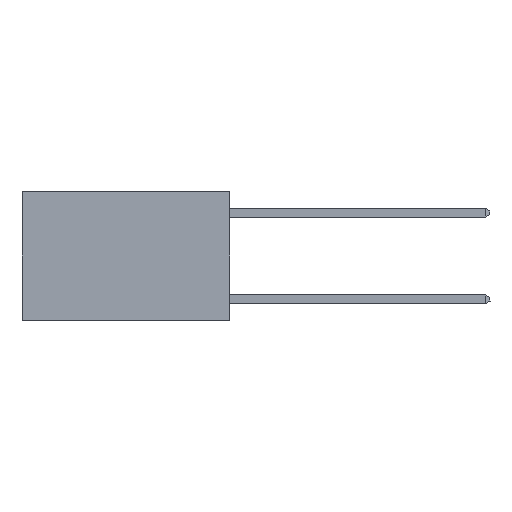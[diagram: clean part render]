
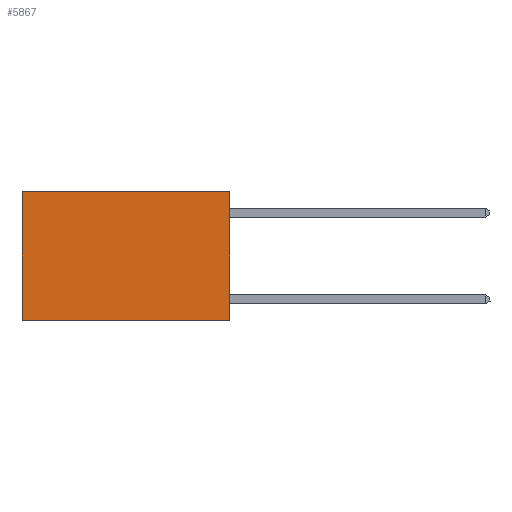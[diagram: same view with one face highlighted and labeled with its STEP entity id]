
A CAD part, left-side view. The second image highlights one B-rep face of the part: STEP entity #5867.
In plain terms, the highlighted planar face has unit normal (-1, 0, 0).
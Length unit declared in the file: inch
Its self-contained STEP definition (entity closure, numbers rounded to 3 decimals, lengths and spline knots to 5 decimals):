
#1160 = CARTESIAN_POINT ( 'NONE',  ( 0.2625, 0.6, -0.37 ) ) ;
#1286 = DIRECTION ( 'NONE',  ( 1., 0., 0. ) ) ;
#1673 = EDGE_CURVE ( 'NONE', #22729, #9185, #2905, .T. ) ;
#2905 = LINE ( 'NONE', #18244, #14675 ) ;
#4361 = DIRECTION ( 'NONE',  ( 0., 1., 0. ) ) ;
#5867 = ADVANCED_FACE ( 'NONE', ( #14102 ), #15345, .F. ) ;
#7933 = ORIENTED_EDGE ( 'NONE', *, *, #1673, .F. ) ;
#8819 = ORIENTED_EDGE ( 'NONE', *, *, #15707, .F. ) ;
#9059 = VERTEX_POINT ( 'NONE', #19527 ) ;
#9185 = VERTEX_POINT ( 'NONE', #1160 ) ;
#11698 = AXIS2_PLACEMENT_3D ( 'NONE', #29335, #1286, #17707 ) ;
#11913 = VERTEX_POINT ( 'NONE', #14825 ) ;
#13159 = VECTOR ( 'NONE', #26403, 39.37008 ) ;
#14102 = FACE_OUTER_BOUND ( 'NONE', #21233, .T. ) ;
#14641 = DIRECTION ( 'NONE',  ( 0., 0., -1. ) ) ;
#14675 = VECTOR ( 'NONE', #18348, 39.37008 ) ;
#14825 = CARTESIAN_POINT ( 'NONE',  ( 0.2625, 0., 0. ) ) ;
#15050 = LINE ( 'NONE', #16110, #26041 ) ;
#15345 = PLANE ( 'NONE',  #11698 ) ;
#15707 = EDGE_CURVE ( 'NONE', #11913, #22729, #19404, .T. ) ;
#16092 = CARTESIAN_POINT ( 'NONE',  ( 0.2625, 0., -0.37 ) ) ;
#16110 = CARTESIAN_POINT ( 'NONE',  ( 0.2625, 0., 0. ) ) ;
#17707 = DIRECTION ( 'NONE',  ( 0., 0., -1. ) ) ;
#18244 = CARTESIAN_POINT ( 'NONE',  ( 0.2625, 0., -0.37 ) ) ;
#18348 = DIRECTION ( 'NONE',  ( 0., 1., 0. ) ) ;
#19404 = LINE ( 'NONE', #21720, #13159 ) ;
#19527 = CARTESIAN_POINT ( 'NONE',  ( 0.2625, 0.6, 0. ) ) ;
#19901 = EDGE_CURVE ( 'NONE', #9059, #9185, #24639, .T. ) ;
#20214 = ORIENTED_EDGE ( 'NONE', *, *, #19901, .T. ) ;
#21097 = ORIENTED_EDGE ( 'NONE', *, *, #26874, .T. ) ;
#21233 = EDGE_LOOP ( 'NONE', ( #20214, #7933, #8819, #21097 ) ) ;
#21720 = CARTESIAN_POINT ( 'NONE',  ( 0.2625, 0., 0. ) ) ;
#22729 = VERTEX_POINT ( 'NONE', #16092 ) ;
#24639 = LINE ( 'NONE', #26317, #30073 ) ;
#26041 = VECTOR ( 'NONE', #4361, 39.37008 ) ;
#26317 = CARTESIAN_POINT ( 'NONE',  ( 0.2625, 0.6, 0. ) ) ;
#26403 = DIRECTION ( 'NONE',  ( 0., 0., -1. ) ) ;
#26874 = EDGE_CURVE ( 'NONE', #11913, #9059, #15050, .T. ) ;
#29335 = CARTESIAN_POINT ( 'NONE',  ( 0.2625, 0., 0. ) ) ;
#30073 = VECTOR ( 'NONE', #14641, 39.37008 ) ;
